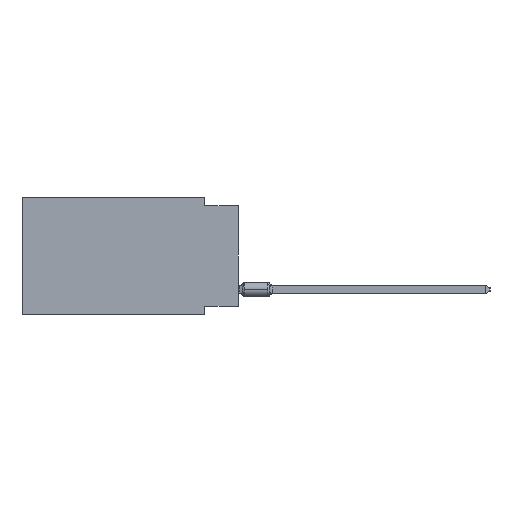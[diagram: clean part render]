
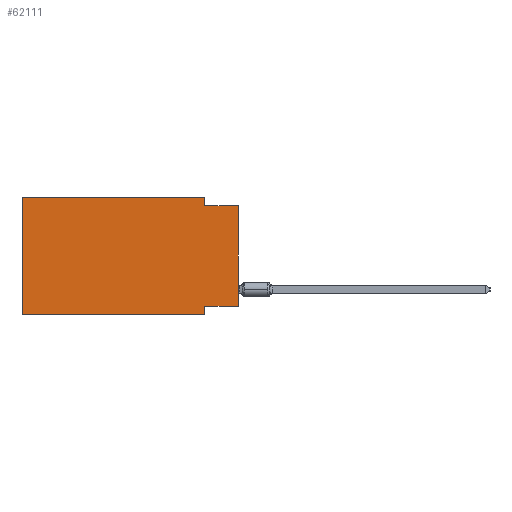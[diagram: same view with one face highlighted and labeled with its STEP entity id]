
A CAD part, left-side view. The second image highlights one B-rep face of the part: STEP entity #62111.
In plain terms, the highlighted planar face has unit normal (-1, 0, 0).
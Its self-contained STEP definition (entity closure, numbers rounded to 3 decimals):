
#3016 = DIRECTION ( 'NONE',  ( 0., -1., 0. ) ) ;
#4059 = EDGE_CURVE ( 'NONE', #22254, #59330, #24392, .T. ) ;
#6180 = LINE ( 'NONE', #41239, #57382 ) ;
#9103 = LINE ( 'NONE', #32331, #71542 ) ;
#10250 = EDGE_CURVE ( 'NONE', #49311, #59330, #70605, .T. ) ;
#11741 = EDGE_CURVE ( 'NONE', #53801, #22254, #69080, .T. ) ;
#14957 = VERTEX_POINT ( 'NONE', #32067 ) ;
#15627 = FACE_OUTER_BOUND ( 'NONE', #36723, .T. ) ;
#17416 = ORIENTED_EDGE ( 'NONE', *, *, #61823, .F. ) ;
#17769 = ORIENTED_EDGE ( 'NONE', *, *, #52240, .F. ) ;
#18340 = DIRECTION ( 'NONE',  ( 0., -1., 0. ) ) ;
#18341 = DIRECTION ( 'NONE',  ( 0., 0., 1. ) ) ;
#19557 = VERTEX_POINT ( 'NONE', #69907 ) ;
#20114 = ORIENTED_EDGE ( 'NONE', *, *, #10250, .T. ) ;
#20520 = CARTESIAN_POINT ( 'NONE',  ( 0., 16.383, 0. ) ) ;
#22254 = VERTEX_POINT ( 'NONE', #23617 ) ;
#22467 = CARTESIAN_POINT ( 'NONE',  ( 0., 16.383, 0. ) ) ;
#23617 = CARTESIAN_POINT ( 'NONE',  ( 0., 2.54, -8.255 ) ) ;
#23702 = VECTOR ( 'NONE', #36225, 1000. ) ;
#24392 = LINE ( 'NONE', #71702, #23702 ) ;
#26719 = CARTESIAN_POINT ( 'NONE',  ( 0., 0., -8.255 ) ) ;
#27415 = PLANE ( 'NONE',  #69413 ) ;
#28894 = ORIENTED_EDGE ( 'NONE', *, *, #53002, .T. ) ;
#29299 = VECTOR ( 'NONE', #43941, 1000. ) ;
#31635 = CARTESIAN_POINT ( 'NONE',  ( 0., 2.54, 0. ) ) ;
#31718 = CARTESIAN_POINT ( 'NONE',  ( 0., 2.54, 0. ) ) ;
#31737 = VECTOR ( 'NONE', #34342, 1000. ) ;
#32067 = CARTESIAN_POINT ( 'NONE',  ( 0., 0., -0.635 ) ) ;
#32331 = CARTESIAN_POINT ( 'NONE',  ( 0., 16.383, 0. ) ) ;
#34342 = DIRECTION ( 'NONE',  ( 0., 1., 0. ) ) ;
#36225 = DIRECTION ( 'NONE',  ( 0., 0., -1. ) ) ;
#36425 = CARTESIAN_POINT ( 'NONE',  ( 0., 2.54, -8.89 ) ) ;
#36723 = EDGE_LOOP ( 'NONE', ( #28894, #43769, #69094, #17769, #17416, #20114, #64340, #74358 ) ) ;
#37533 = VECTOR ( 'NONE', #66507, 1000. ) ;
#41239 = CARTESIAN_POINT ( 'NONE',  ( 0., 16.383, 0. ) ) ;
#42481 = CARTESIAN_POINT ( 'NONE',  ( 0., 0., 0. ) ) ;
#43769 = ORIENTED_EDGE ( 'NONE', *, *, #65757, .F. ) ;
#43941 = DIRECTION ( 'NONE',  ( 0., 0., -1. ) ) ;
#45792 = CARTESIAN_POINT ( 'NONE',  ( 0., 16.383, -8.89 ) ) ;
#46579 = CARTESIAN_POINT ( 'NONE',  ( 0., 16.383, -8.89 ) ) ;
#49311 = VERTEX_POINT ( 'NONE', #45792 ) ;
#52240 = EDGE_CURVE ( 'NONE', #67583, #61997, #9103, .T. ) ;
#53002 = EDGE_CURVE ( 'NONE', #53801, #14957, #66884, .T. ) ;
#53801 = VERTEX_POINT ( 'NONE', #26719 ) ;
#54042 = VECTOR ( 'NONE', #59936, 1000. ) ;
#54755 = VECTOR ( 'NONE', #18340, 1000. ) ;
#56090 = EDGE_CURVE ( 'NONE', #61997, #19557, #67972, .T. ) ;
#57382 = VECTOR ( 'NONE', #18341, 1000. ) ;
#59330 = VERTEX_POINT ( 'NONE', #36425 ) ;
#59936 = DIRECTION ( 'NONE',  ( 0., -1., 0. ) ) ;
#61068 = CARTESIAN_POINT ( 'NONE',  ( 0., 0., -0.635 ) ) ;
#61823 = EDGE_CURVE ( 'NONE', #49311, #67583, #6180, .T. ) ;
#61997 = VERTEX_POINT ( 'NONE', #31635 ) ;
#62111 = ADVANCED_FACE ( 'NONE', ( #15627 ), #27415, .F. ) ;
#63294 = DIRECTION ( 'NONE',  ( 0., 0., -1. ) ) ;
#63349 = CARTESIAN_POINT ( 'NONE',  ( 0., 0., -8.255 ) ) ;
#64340 = ORIENTED_EDGE ( 'NONE', *, *, #4059, .F. ) ;
#65757 = EDGE_CURVE ( 'NONE', #19557, #14957, #72124, .T. ) ;
#66507 = DIRECTION ( 'NONE',  ( 0., 0., 1. ) ) ;
#66884 = LINE ( 'NONE', #42481, #37533 ) ;
#67583 = VERTEX_POINT ( 'NONE', #20520 ) ;
#67972 = LINE ( 'NONE', #31718, #29299 ) ;
#69080 = LINE ( 'NONE', #63349, #31737 ) ;
#69094 = ORIENTED_EDGE ( 'NONE', *, *, #56090, .F. ) ;
#69394 = DIRECTION ( 'NONE',  ( 1., 0., 0. ) ) ;
#69413 = AXIS2_PLACEMENT_3D ( 'NONE', #22467, #69394, #63294 ) ;
#69907 = CARTESIAN_POINT ( 'NONE',  ( 0., 2.54, -0.635 ) ) ;
#70605 = LINE ( 'NONE', #46579, #54755 ) ;
#71542 = VECTOR ( 'NONE', #3016, 1000. ) ;
#71702 = CARTESIAN_POINT ( 'NONE',  ( 0., 2.54, -8.89 ) ) ;
#72124 = LINE ( 'NONE', #61068, #54042 ) ;
#74358 = ORIENTED_EDGE ( 'NONE', *, *, #11741, .F. ) ;
